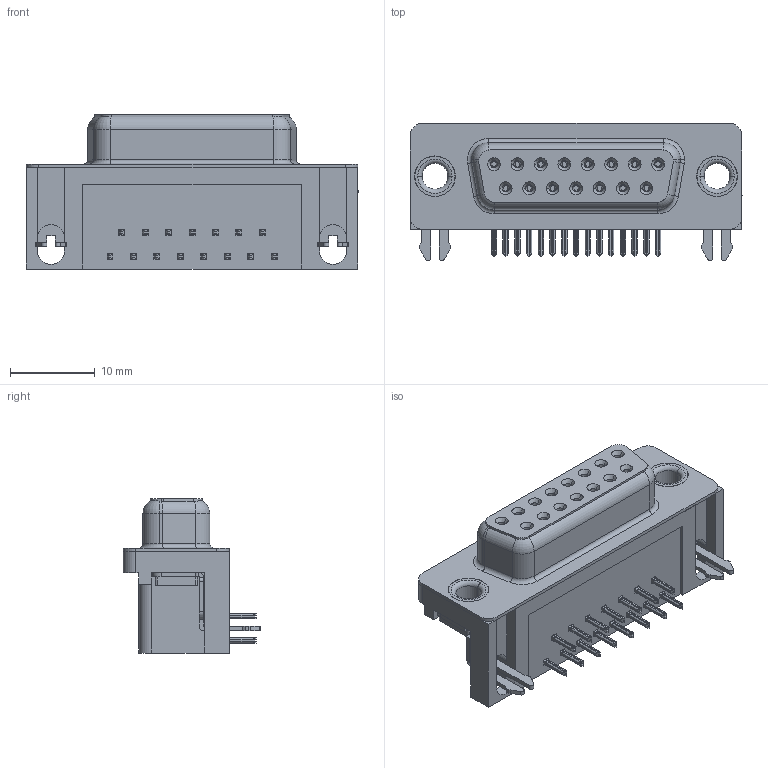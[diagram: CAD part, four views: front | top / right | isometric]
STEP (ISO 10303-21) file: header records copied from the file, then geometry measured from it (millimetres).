
FILE_DESCRIPTION (( 'STEP AP203' ), '1' );
FILE_NAME ('622-015-668-531.STEP', '2019-11-20T01:37:35', ( '' ), ( '' ), 'SwSTEP 2.0', 'SolidWorks 2016', '' );
FILE_SCHEMA (( 'CONFIG_CONTROL_DESIGN' ));
Length unit declared in the file: millimetre
Products named in the file (7): 622 Housing_15 Socket; 622 Contact Top; 622 Shell_15 Socket; 622-015-668-531; 622 Socket Bottom; 622 Thru Hole Rivet; 622 2 Prong Board Lock
Assembly tree (21 placements, depth 2):
  622-015-668-531
    622 Housing_15 Socket
    622 Shell_15 Socket
    622 Socket Bottom  x7
    622 Contact Top  x8
    622 2 Prong Board Lock  x2
    622 Thru Hole Rivet  x2
Bounding box: 39.22 x 16.25 x 18.2 mm (x, y, z)
Volume: 5175 mm3; surface area: 6697.9 mm2
Topology: 21 solids, 21 shells, 2427 faces, 6378 edges, 4008 vertices
Faces by surface type: plane 1106, cylinder 595, bspline 512, cone 180, torus 34
Entity records: 24884 total; most frequent: CARTESIAN_POINT 7255, ORIENTED_EDGE 3546, DIRECTION 3204, EDGE_CURVE 1773, VERTEX_POINT 1130, VECTOR 1124, LINE 1124, AXIS2_PLACEMENT_3D 1040
